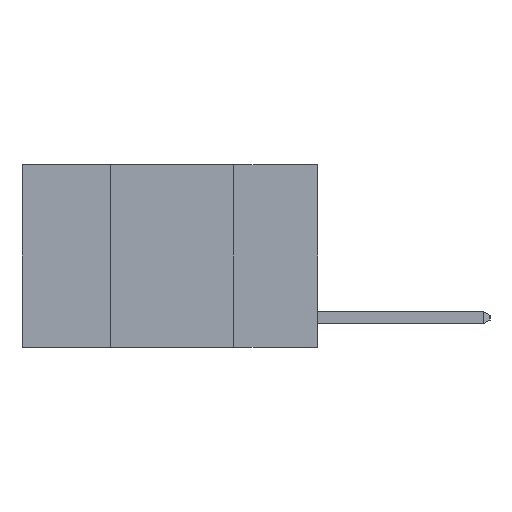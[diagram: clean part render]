
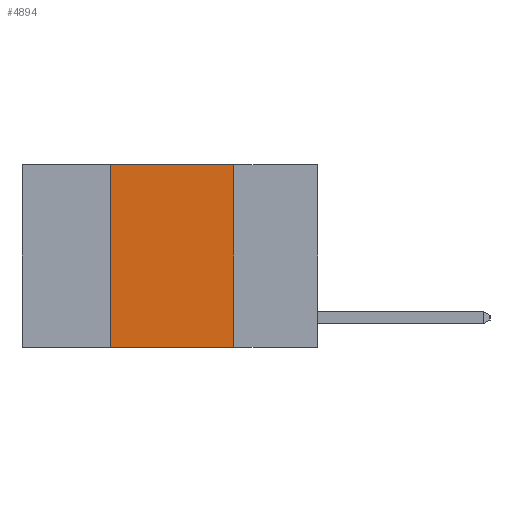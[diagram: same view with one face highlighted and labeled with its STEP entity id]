
A CAD part, left-side view. The second image highlights one B-rep face of the part: STEP entity #4894.
In plain terms, the highlighted planar face has unit normal (-1, 0, 0).
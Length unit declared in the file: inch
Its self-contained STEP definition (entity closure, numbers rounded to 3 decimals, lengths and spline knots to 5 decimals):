
#114 = EDGE_CURVE ( 'NONE', #3342, #5498, #9335, .T. ) ;
#301 = ORIENTED_EDGE ( 'NONE', *, *, #6997, .F. ) ;
#539 = DIRECTION ( 'NONE',  ( 0., 0., 1. ) ) ;
#976 = DIRECTION ( 'NONE',  ( 1., 0., 0. ) ) ;
#1024 = EDGE_CURVE ( 'NONE', #3342, #2011, #11733, .T. ) ;
#1595 = LINE ( 'NONE', #7204, #8453 ) ;
#2010 = CARTESIAN_POINT ( 'NONE',  ( 0., 0.6, 0. ) ) ;
#2011 = VERTEX_POINT ( 'NONE', #7614 ) ;
#3321 = VECTOR ( 'NONE', #539, 39.37008 ) ;
#3342 = VERTEX_POINT ( 'NONE', #8071 ) ;
#4639 = CARTESIAN_POINT ( 'NONE',  ( 0., 0.17, 0. ) ) ;
#4894 = ADVANCED_FACE ( 'NONE', ( #9573 ), #15326, .F. ) ;
#5498 = VERTEX_POINT ( 'NONE', #8178 ) ;
#5750 = DIRECTION ( 'NONE',  ( 0., -1., 0. ) ) ;
#5905 = AXIS2_PLACEMENT_3D ( 'NONE', #7053, #976, #9419 ) ;
#6027 = ORIENTED_EDGE ( 'NONE', *, *, #9951, .F. ) ;
#6268 = EDGE_LOOP ( 'NONE', ( #6027, #301, #6776, #7149 ) ) ;
#6776 = ORIENTED_EDGE ( 'NONE', *, *, #114, .F. ) ;
#6997 = EDGE_CURVE ( 'NONE', #5498, #7052, #13410, .T. ) ;
#7052 = VERTEX_POINT ( 'NONE', #4639 ) ;
#7053 = CARTESIAN_POINT ( 'NONE',  ( 0., 0.6, 0. ) ) ;
#7149 = ORIENTED_EDGE ( 'NONE', *, *, #1024, .T. ) ;
#7204 = CARTESIAN_POINT ( 'NONE',  ( 0., 0.17, 0. ) ) ;
#7614 = CARTESIAN_POINT ( 'NONE',  ( 0., 0.17, -0.37 ) ) ;
#8071 = CARTESIAN_POINT ( 'NONE',  ( 0., 0.42, -0.37 ) ) ;
#8178 = CARTESIAN_POINT ( 'NONE',  ( 0., 0.42, 0. ) ) ;
#8453 = VECTOR ( 'NONE', #15482, 39.37008 ) ;
#9335 = LINE ( 'NONE', #12354, #3321 ) ;
#9419 = DIRECTION ( 'NONE',  ( 0., 0., -1. ) ) ;
#9573 = FACE_OUTER_BOUND ( 'NONE', #6268, .T. ) ;
#9951 = EDGE_CURVE ( 'NONE', #7052, #2011, #1595, .T. ) ;
#10240 = VECTOR ( 'NONE', #5750, 39.37008 ) ;
#11733 = LINE ( 'NONE', #12093, #12115 ) ;
#12093 = CARTESIAN_POINT ( 'NONE',  ( 0., 0.6, -0.37 ) ) ;
#12115 = VECTOR ( 'NONE', #12794, 39.37008 ) ;
#12354 = CARTESIAN_POINT ( 'NONE',  ( 0., 0.42, 0. ) ) ;
#12794 = DIRECTION ( 'NONE',  ( 0., -1., 0. ) ) ;
#13410 = LINE ( 'NONE', #2010, #10240 ) ;
#15326 = PLANE ( 'NONE',  #5905 ) ;
#15482 = DIRECTION ( 'NONE',  ( 0., 0., -1. ) ) ;
